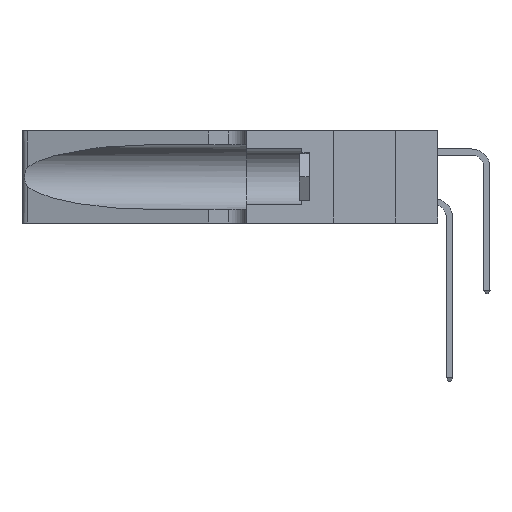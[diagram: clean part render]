
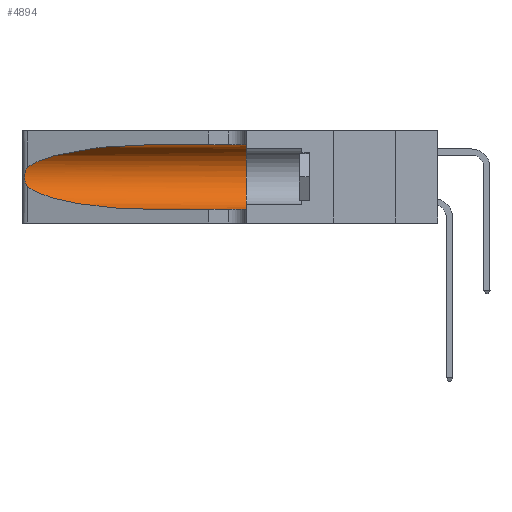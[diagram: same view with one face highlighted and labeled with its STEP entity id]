
A CAD part, left-side view. The second image highlights one B-rep face of the part: STEP entity #4894.
In plain terms, the highlighted cylindrical face has radius 3.308 mm (diameter 6.617 mm), a partial arc.
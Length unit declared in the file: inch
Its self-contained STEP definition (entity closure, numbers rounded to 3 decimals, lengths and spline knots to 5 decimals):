
#153 = CARTESIAN_POINT ( 'NONE',  ( 0.1305, 0.35, 0.31525 ) ) ;
#375 = VECTOR ( 'NONE', #31402, 39.37008 ) ;
#968 = CARTESIAN_POINT ( 'NONE',  ( 0.25854, 1.2359, 0.20912 ) ) ;
#1094 = CARTESIAN_POINT ( 'NONE',  ( 0.25639, 1.23186, 0.15144 ) ) ;
#3350 = ORIENTED_EDGE ( 'NONE', *, *, #33152, .T. ) ;
#3804 = CARTESIAN_POINT ( 'NONE',  ( 0.25555, 1.22994, 0.2215 ) ) ;
#3933 = CARTESIAN_POINT ( 'NONE',  ( 0.25555, 1.22993, 0.14849 ) ) ;
#4894 = ADVANCED_FACE ( 'NONE', ( #20972 ), #5265, .F. ) ;
#5203 = CARTESIAN_POINT ( 'NONE',  ( 0.25487, 1.22718, 0.22369 ) ) ;
#5265 = CYLINDRICAL_SURFACE ( 'NONE', #31625, 0.13025 ) ;
#5646 = CARTESIAN_POINT ( 'NONE',  ( 0.1305, 0.72297, 0.05475 ) ) ;
#6586 = CARTESIAN_POINT ( 'NONE',  ( 0.25487, 1.22718, 0.14631 ) ) ;
#6784 = CARTESIAN_POINT ( 'NONE',  ( 0.25789, 1.23486, 0.15765 ) ) ;
#7024 = AXIS2_PLACEMENT_3D ( 'NONE', #26265, #35304, #8454 ) ;
#7238 =( BOUNDED_CURVE ( )  B_SPLINE_CURVE ( 3, ( #6586, #27253, #10566, #5646 ),
 .UNSPECIFIED., .F., .F. ) 
 B_SPLINE_CURVE_WITH_KNOTS ( ( 4, 4 ),
 ( 3.44316, 4.71239 ),
 .UNSPECIFIED. ) 
 CURVE ( )  GEOMETRIC_REPRESENTATION_ITEM ( )  RATIONAL_B_SPLINE_CURVE ( ( 1., 0.87, 0.87, 1. ) ) 
 REPRESENTATION_ITEM ( '' )  );
#7465 = B_SPLINE_CURVE_WITH_KNOTS ( 'NONE', 3,
 ( #15812, #3804, #24584, #24965, #968, #13222, #16170, #27697, #36473, #30812, #6784, #1094, #3933, #21501 ),
 .UNSPECIFIED., .F., .F.,
 ( 4, 2, 2, 2, 2, 2, 4 ),
 ( 0., 0.00027, 0.00053, 0.00107, 0.0016, 0.00187, 0.00214 ),
 .UNSPECIFIED. ) ;
#7905 = VERTEX_POINT ( 'NONE', #33669 ) ;
#8130 = CARTESIAN_POINT ( 'NONE',  ( 0.18966, 0.96281, 0.31525 ) ) ;
#8362 = VERTEX_POINT ( 'NONE', #15477 ) ;
#8454 = DIRECTION ( 'NONE',  ( 0., 0., 1. ) ) ;
#9882 = CARTESIAN_POINT ( 'NONE',  ( 0.1305, 0.35, 0.05475 ) ) ;
#9958 = EDGE_CURVE ( 'NONE', #8362, #7905, #7238, .T. ) ;
#10566 = CARTESIAN_POINT ( 'NONE',  ( 0.18966, 0.96281, 0.05475 ) ) ;
#10606 = EDGE_CURVE ( 'NONE', #14093, #25176, #18104, .T. ) ;
#10650 = CARTESIAN_POINT ( 'NONE',  ( 0.1305, 1.61858, 0.31525 ) ) ;
#11929 = ORIENTED_EDGE ( 'NONE', *, *, #19390, .T. ) ;
#13222 = CARTESIAN_POINT ( 'NONE',  ( 0.26018, 1.23835, 0.19895 ) ) ;
#14093 = VERTEX_POINT ( 'NONE', #34260 ) ;
#15477 = CARTESIAN_POINT ( 'NONE',  ( 0.25487, 1.22718, 0.14631 ) ) ;
#15812 = CARTESIAN_POINT ( 'NONE',  ( 0.25487, 1.22718, 0.22369 ) ) ;
#16170 = CARTESIAN_POINT ( 'NONE',  ( 0.26075, 1.23896, 0.19203 ) ) ;
#16185 = ORIENTED_EDGE ( 'NONE', *, *, #9958, .T. ) ;
#17602 = VECTOR ( 'NONE', #31198, 39.37008 ) ;
#18104 =( BOUNDED_CURVE ( )  B_SPLINE_CURVE ( 3, ( #25813, #8130, #34121, #25309 ),
 .UNSPECIFIED., .F., .T. ) 
 B_SPLINE_CURVE_WITH_KNOTS ( ( 4, 4 ),
 ( 1.5708, 2.84003 ),
 .UNSPECIFIED. ) 
 CURVE ( )  GEOMETRIC_REPRESENTATION_ITEM ( )  RATIONAL_B_SPLINE_CURVE ( ( 1., 0.87, 0.87, 1. ) ) 
 REPRESENTATION_ITEM ( '' )  );
#19390 = EDGE_CURVE ( 'NONE', #25176, #8362, #7465, .T. ) ;
#20390 = LINE ( 'NONE', #10650, #17602 ) ;
#20972 = FACE_OUTER_BOUND ( 'NONE', #24323, .T. ) ;
#21501 = CARTESIAN_POINT ( 'NONE',  ( 0.25487, 1.22718, 0.14631 ) ) ;
#22868 = DIRECTION ( 'NONE',  ( 0., 0., -1. ) ) ;
#23327 = EDGE_CURVE ( 'NONE', #30736, #31997, #25941, .T. ) ;
#24323 = EDGE_LOOP ( 'NONE', ( #24549, #11929, #16185, #3350, #31366, #30972 ) ) ;
#24549 = ORIENTED_EDGE ( 'NONE', *, *, #10606, .T. ) ;
#24584 = CARTESIAN_POINT ( 'NONE',  ( 0.25639, 1.23184, 0.21858 ) ) ;
#24965 = CARTESIAN_POINT ( 'NONE',  ( 0.25787, 1.23484, 0.2124 ) ) ;
#25176 = VERTEX_POINT ( 'NONE', #5203 ) ;
#25309 = CARTESIAN_POINT ( 'NONE',  ( 0.25487, 1.22718, 0.22369 ) ) ;
#25813 = CARTESIAN_POINT ( 'NONE',  ( 0.1305, 0.72297, 0.31525 ) ) ;
#25941 = CIRCLE ( 'NONE', #7024, 0.13025 ) ;
#26265 = CARTESIAN_POINT ( 'NONE',  ( 0.1305, 0.35, 0.185 ) ) ;
#26289 = EDGE_CURVE ( 'NONE', #14093, #30736, #20390, .T. ) ;
#27152 = DIRECTION ( 'NONE',  ( 0., -1., 0. ) ) ;
#27253 = CARTESIAN_POINT ( 'NONE',  ( 0.2373, 1.15595, 0.08982 ) ) ;
#27697 = CARTESIAN_POINT ( 'NONE',  ( 0.26075, 1.23896, 0.178 ) ) ;
#29035 = LINE ( 'NONE', #36573, #375 ) ;
#30736 = VERTEX_POINT ( 'NONE', #153 ) ;
#30812 = CARTESIAN_POINT ( 'NONE',  ( 0.25856, 1.23593, 0.16098 ) ) ;
#30865 = CARTESIAN_POINT ( 'NONE',  ( 0.1305, 1.61858, 0.185 ) ) ;
#30972 = ORIENTED_EDGE ( 'NONE', *, *, #26289, .F. ) ;
#31198 = DIRECTION ( 'NONE',  ( 0., -1., 0. ) ) ;
#31366 = ORIENTED_EDGE ( 'NONE', *, *, #23327, .F. ) ;
#31402 = DIRECTION ( 'NONE',  ( 0., -1., 0. ) ) ;
#31625 = AXIS2_PLACEMENT_3D ( 'NONE', #30865, #27152, #22868 ) ;
#31997 = VERTEX_POINT ( 'NONE', #9882 ) ;
#33152 = EDGE_CURVE ( 'NONE', #7905, #31997, #29035, .T. ) ;
#33669 = CARTESIAN_POINT ( 'NONE',  ( 0.1305, 0.72297, 0.05475 ) ) ;
#34121 = CARTESIAN_POINT ( 'NONE',  ( 0.2373, 1.15595, 0.28018 ) ) ;
#34260 = CARTESIAN_POINT ( 'NONE',  ( 0.1305, 0.72297, 0.31525 ) ) ;
#35304 = DIRECTION ( 'NONE',  ( 0., 1., 0. ) ) ;
#36473 = CARTESIAN_POINT ( 'NONE',  ( 0.26017, 1.23833, 0.17102 ) ) ;
#36573 = CARTESIAN_POINT ( 'NONE',  ( 0.1305, 1.61858, 0.05475 ) ) ;
